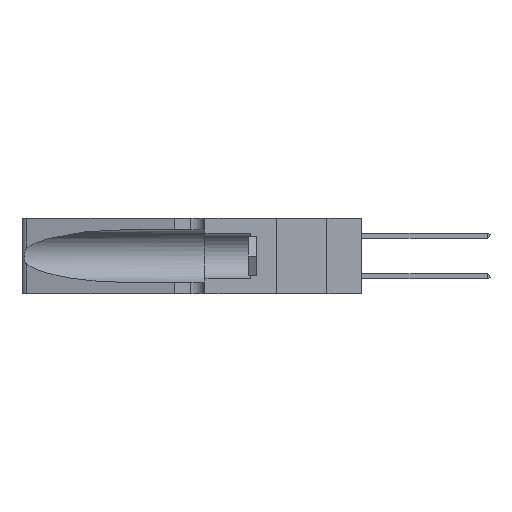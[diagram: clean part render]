
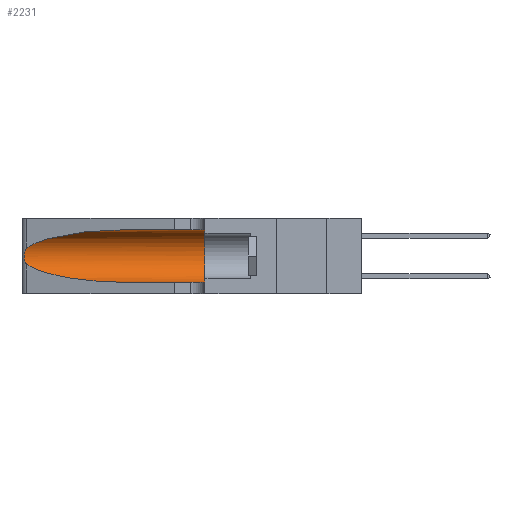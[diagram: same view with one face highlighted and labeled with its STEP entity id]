
A CAD part, left-side view. The second image highlights one B-rep face of the part: STEP entity #2231.
In plain terms, the highlighted cylindrical face has radius 3.308 mm (diameter 6.617 mm), a partial arc.
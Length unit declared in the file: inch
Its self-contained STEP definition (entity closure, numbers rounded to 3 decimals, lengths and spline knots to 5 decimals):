
#55 = VERTEX_POINT ( 'NONE', #8783 ) ;
#506 = CARTESIAN_POINT ( 'NONE',  ( 0.1305, 0.72297, 0.05475 ) ) ;
#1042 = CARTESIAN_POINT ( 'NONE',  ( 0.1305, 0.72297, 0.31525 ) ) ;
#1279 = CARTESIAN_POINT ( 'NONE',  ( 0.25555, 1.22994, 0.2215 ) ) ;
#1373 = ORIENTED_EDGE ( 'NONE', *, *, #15141, .T. ) ;
#1395 = CARTESIAN_POINT ( 'NONE',  ( 0.25555, 1.22993, 0.14849 ) ) ;
#1422 = ORIENTED_EDGE ( 'NONE', *, *, #14549, .F. ) ;
#1976 = LINE ( 'NONE', #19639, #28575 ) ;
#2231 = ADVANCED_FACE ( 'NONE', ( #4739 ), #23666, .F. ) ;
#2524 = CARTESIAN_POINT ( 'NONE',  ( 0.18966, 0.96281, 0.05475 ) ) ;
#2662 = EDGE_CURVE ( 'NONE', #14886, #11045, #17645, .T. ) ;
#3020 = CARTESIAN_POINT ( 'NONE',  ( 0.1305, 1.61858, 0.185 ) ) ;
#4154 = DIRECTION ( 'NONE',  ( 0., -1., 0. ) ) ;
#4739 = FACE_OUTER_BOUND ( 'NONE', #18912, .T. ) ;
#6072 = LINE ( 'NONE', #32231, #6884 ) ;
#6520 = CARTESIAN_POINT ( 'NONE',  ( 0.25787, 1.23484, 0.2124 ) ) ;
#6884 = VECTOR ( 'NONE', #14400, 39.37008 ) ;
#7286 = DIRECTION ( 'NONE',  ( 0., 1., 0. ) ) ;
#8783 = CARTESIAN_POINT ( 'NONE',  ( 0.25487, 1.22718, 0.22369 ) ) ;
#9114 = CARTESIAN_POINT ( 'NONE',  ( 0.26018, 1.23835, 0.19895 ) ) ;
#9500 =( BOUNDED_CURVE ( )  B_SPLINE_CURVE ( 3, ( #15458, #18020, #2524, #20605 ),
 .UNSPECIFIED., .F., .F. ) 
 B_SPLINE_CURVE_WITH_KNOTS ( ( 4, 4 ),
 ( 3.44316, 4.71239 ),
 .UNSPECIFIED. ) 
 CURVE ( )  GEOMETRIC_REPRESENTATION_ITEM ( )  RATIONAL_B_SPLINE_CURVE ( ( 1., 0.87, 0.87, 1. ) ) 
 REPRESENTATION_ITEM ( '' )  );
#9874 = CARTESIAN_POINT ( 'NONE',  ( 0.18966, 0.96281, 0.31525 ) ) ;
#11045 = VERTEX_POINT ( 'NONE', #28913 ) ;
#11760 = CARTESIAN_POINT ( 'NONE',  ( 0.26075, 1.23896, 0.178 ) ) ;
#12672 = EDGE_CURVE ( 'NONE', #27105, #55, #13073, .T. ) ;
#13073 =( BOUNDED_CURVE ( )  B_SPLINE_CURVE ( 3, ( #27830, #9874, #15092, #32931 ),
 .UNSPECIFIED., .F., .T. ) 
 B_SPLINE_CURVE_WITH_KNOTS ( ( 4, 4 ),
 ( 1.5708, 2.84003 ),
 .UNSPECIFIED. ) 
 CURVE ( )  GEOMETRIC_REPRESENTATION_ITEM ( )  RATIONAL_B_SPLINE_CURVE ( ( 1., 0.87, 0.87, 1. ) ) 
 REPRESENTATION_ITEM ( '' )  );
#13492 = CARTESIAN_POINT ( 'NONE',  ( 0.1305, 0.35, 0.31525 ) ) ;
#14376 = CARTESIAN_POINT ( 'NONE',  ( 0.25856, 1.23593, 0.16098 ) ) ;
#14400 = DIRECTION ( 'NONE',  ( 0., -1., 0. ) ) ;
#14489 = ORIENTED_EDGE ( 'NONE', *, *, #2662, .F. ) ;
#14549 = EDGE_CURVE ( 'NONE', #27105, #14886, #6072, .T. ) ;
#14886 = VERTEX_POINT ( 'NONE', #13492 ) ;
#15091 = EDGE_CURVE ( 'NONE', #55, #23682, #24967, .T. ) ;
#15092 = CARTESIAN_POINT ( 'NONE',  ( 0.2373, 1.15595, 0.28018 ) ) ;
#15141 = EDGE_CURVE ( 'NONE', #22979, #11045, #1976, .T. ) ;
#15458 = CARTESIAN_POINT ( 'NONE',  ( 0.25487, 1.22718, 0.14631 ) ) ;
#16384 = CARTESIAN_POINT ( 'NONE',  ( 0.25487, 1.22718, 0.14631 ) ) ;
#16949 = CARTESIAN_POINT ( 'NONE',  ( 0.25639, 1.23186, 0.15144 ) ) ;
#17645 = CIRCLE ( 'NONE', #27901, 0.13025 ) ;
#18020 = CARTESIAN_POINT ( 'NONE',  ( 0.2373, 1.15595, 0.08982 ) ) ;
#18531 = DIRECTION ( 'NONE',  ( 0., 0., -1. ) ) ;
#18912 = EDGE_LOOP ( 'NONE', ( #29762, #28254, #23497, #1373, #14489, #1422 ) ) ;
#19525 = CARTESIAN_POINT ( 'NONE',  ( 0.25487, 1.22718, 0.14631 ) ) ;
#19639 = CARTESIAN_POINT ( 'NONE',  ( 0.1305, 1.61858, 0.05475 ) ) ;
#19862 = EDGE_CURVE ( 'NONE', #23682, #22979, #9500, .T. ) ;
#20605 = CARTESIAN_POINT ( 'NONE',  ( 0.1305, 0.72297, 0.05475 ) ) ;
#21964 = CARTESIAN_POINT ( 'NONE',  ( 0.25639, 1.23184, 0.21858 ) ) ;
#22748 = CARTESIAN_POINT ( 'NONE',  ( 0.1305, 0.35, 0.185 ) ) ;
#22979 = VERTEX_POINT ( 'NONE', #506 ) ;
#23497 = ORIENTED_EDGE ( 'NONE', *, *, #19862, .T. ) ;
#23649 = DIRECTION ( 'NONE',  ( 0., -1., 0. ) ) ;
#23666 = CYLINDRICAL_SURFACE ( 'NONE', #28088, 0.13025 ) ;
#23682 = VERTEX_POINT ( 'NONE', #16384 ) ;
#24546 = CARTESIAN_POINT ( 'NONE',  ( 0.25854, 1.2359, 0.20912 ) ) ;
#24967 = B_SPLINE_CURVE_WITH_KNOTS ( 'NONE', 3,
 ( #32099, #1279, #21964, #6520, #24546, #9114, #27114, #11760, #29675, #14376, #32203, #16949, #1395, #19525 ),
 .UNSPECIFIED., .F., .F.,
 ( 4, 2, 2, 2, 2, 2, 4 ),
 ( 0., 0.00027, 0.00053, 0.00107, 0.0016, 0.00187, 0.00214 ),
 .UNSPECIFIED. ) ;
#25316 = DIRECTION ( 'NONE',  ( 0., 0., 1. ) ) ;
#27105 = VERTEX_POINT ( 'NONE', #1042 ) ;
#27114 = CARTESIAN_POINT ( 'NONE',  ( 0.26075, 1.23896, 0.19203 ) ) ;
#27830 = CARTESIAN_POINT ( 'NONE',  ( 0.1305, 0.72297, 0.31525 ) ) ;
#27901 = AXIS2_PLACEMENT_3D ( 'NONE', #22748, #7286, #25316 ) ;
#28088 = AXIS2_PLACEMENT_3D ( 'NONE', #3020, #23649, #18531 ) ;
#28254 = ORIENTED_EDGE ( 'NONE', *, *, #15091, .T. ) ;
#28575 = VECTOR ( 'NONE', #4154, 39.37008 ) ;
#28913 = CARTESIAN_POINT ( 'NONE',  ( 0.1305, 0.35, 0.05475 ) ) ;
#29675 = CARTESIAN_POINT ( 'NONE',  ( 0.26017, 1.23833, 0.17102 ) ) ;
#29762 = ORIENTED_EDGE ( 'NONE', *, *, #12672, .T. ) ;
#32099 = CARTESIAN_POINT ( 'NONE',  ( 0.25487, 1.22718, 0.22369 ) ) ;
#32203 = CARTESIAN_POINT ( 'NONE',  ( 0.25789, 1.23486, 0.15765 ) ) ;
#32231 = CARTESIAN_POINT ( 'NONE',  ( 0.1305, 1.61858, 0.31525 ) ) ;
#32931 = CARTESIAN_POINT ( 'NONE',  ( 0.25487, 1.22718, 0.22369 ) ) ;
